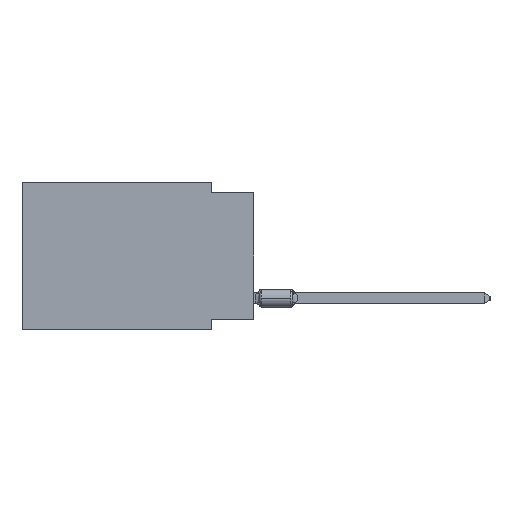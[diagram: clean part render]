
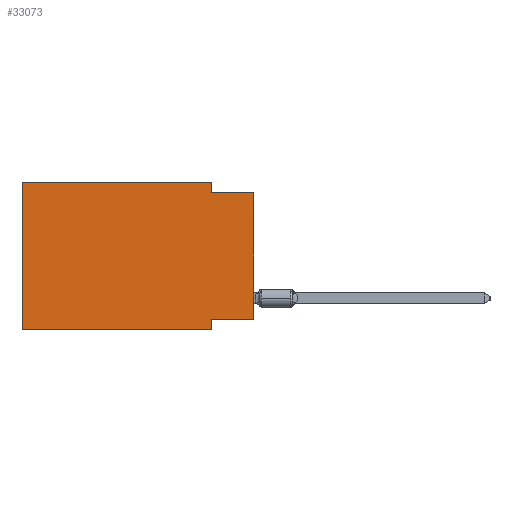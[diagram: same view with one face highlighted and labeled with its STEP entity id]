
A CAD part, left-side view. The second image highlights one B-rep face of the part: STEP entity #33073.
In plain terms, the highlighted planar face has unit normal (-1, 0, 0).
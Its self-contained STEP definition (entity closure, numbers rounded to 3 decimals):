
#757 = DIRECTION ( 'NONE',  ( 0., -1., 0. ) ) ;
#990 = CARTESIAN_POINT ( 'NONE',  ( 0., 0., -0.635 ) ) ;
#1292 = ORIENTED_EDGE ( 'NONE', *, *, #31722, .F. ) ;
#3122 = CARTESIAN_POINT ( 'NONE',  ( 0., 13.97, 0. ) ) ;
#3251 = DIRECTION ( 'NONE',  ( 0., 0., -1. ) ) ;
#3749 = VECTOR ( 'NONE', #3251, 1000. ) ;
#4054 = DIRECTION ( 'NONE',  ( 0., 0., 1. ) ) ;
#5217 = DIRECTION ( 'NONE',  ( 0., -1., 0. ) ) ;
#5792 = DIRECTION ( 'NONE',  ( 0., 0., -1. ) ) ;
#6641 = LINE ( 'NONE', #9706, #14677 ) ;
#6836 = CARTESIAN_POINT ( 'NONE',  ( 0., 2.54, 0. ) ) ;
#6910 = VERTEX_POINT ( 'NONE', #21703 ) ;
#7301 = DIRECTION ( 'NONE',  ( 0., 0., -1. ) ) ;
#7713 = CARTESIAN_POINT ( 'NONE',  ( 0., 2.54, -8.89 ) ) ;
#8044 = EDGE_CURVE ( 'NONE', #12465, #13004, #29062, .T. ) ;
#8526 = DIRECTION ( 'NONE',  ( 0., -1., 0. ) ) ;
#9296 = VECTOR ( 'NONE', #757, 1000. ) ;
#9335 = CARTESIAN_POINT ( 'NONE',  ( 0., 13.97, 0. ) ) ;
#9338 = VERTEX_POINT ( 'NONE', #39653 ) ;
#9567 = CARTESIAN_POINT ( 'NONE',  ( 0., 2.54, 0. ) ) ;
#9706 = CARTESIAN_POINT ( 'NONE',  ( 0., 0., -8.255 ) ) ;
#11923 = ORIENTED_EDGE ( 'NONE', *, *, #25752, .F. ) ;
#12383 = ORIENTED_EDGE ( 'NONE', *, *, #12802, .F. ) ;
#12465 = VERTEX_POINT ( 'NONE', #39825 ) ;
#12802 = EDGE_CURVE ( 'NONE', #9338, #14344, #18124, .T. ) ;
#13004 = VERTEX_POINT ( 'NONE', #26580 ) ;
#14344 = VERTEX_POINT ( 'NONE', #19650 ) ;
#14677 = VECTOR ( 'NONE', #27879, 1000. ) ;
#14922 = VECTOR ( 'NONE', #4054, 1000. ) ;
#15615 = CARTESIAN_POINT ( 'NONE',  ( 0., 13.97, -8.89 ) ) ;
#17947 = ORIENTED_EDGE ( 'NONE', *, *, #23432, .F. ) ;
#18124 = LINE ( 'NONE', #7713, #3749 ) ;
#18371 = ORIENTED_EDGE ( 'NONE', *, *, #41798, .F. ) ;
#19650 = CARTESIAN_POINT ( 'NONE',  ( 0., 2.54, -8.89 ) ) ;
#20772 = AXIS2_PLACEMENT_3D ( 'NONE', #9335, #37853, #5792 ) ;
#21625 = VECTOR ( 'NONE', #5217, 1000. ) ;
#21703 = CARTESIAN_POINT ( 'NONE',  ( 0., 0., -0.635 ) ) ;
#21821 = CARTESIAN_POINT ( 'NONE',  ( 0., 2.54, -0.635 ) ) ;
#21951 = EDGE_CURVE ( 'NONE', #42552, #6910, #26047, .T. ) ;
#22240 = LINE ( 'NONE', #15615, #9296 ) ;
#23432 = EDGE_CURVE ( 'NONE', #40999, #6910, #32838, .T. ) ;
#25019 = VERTEX_POINT ( 'NONE', #9567 ) ;
#25240 = LINE ( 'NONE', #6836, #35665 ) ;
#25752 = EDGE_CURVE ( 'NONE', #13004, #25019, #34215, .T. ) ;
#26047 = LINE ( 'NONE', #44627, #27289 ) ;
#26580 = CARTESIAN_POINT ( 'NONE',  ( 0., 13.97, 0. ) ) ;
#26696 = ORIENTED_EDGE ( 'NONE', *, *, #45926, .T. ) ;
#26736 = DIRECTION ( 'NONE',  ( 0., 0., 1. ) ) ;
#27162 = CARTESIAN_POINT ( 'NONE',  ( 0., 13.97, 0. ) ) ;
#27289 = VECTOR ( 'NONE', #26736, 1000. ) ;
#27879 = DIRECTION ( 'NONE',  ( 0., 1., 0. ) ) ;
#28379 = CARTESIAN_POINT ( 'NONE',  ( 0., 0., -8.255 ) ) ;
#29062 = LINE ( 'NONE', #3122, #14922 ) ;
#30347 = FACE_OUTER_BOUND ( 'NONE', #41518, .T. ) ;
#30799 = PLANE ( 'NONE',  #20772 ) ;
#31165 = VECTOR ( 'NONE', #8526, 1000. ) ;
#31722 = EDGE_CURVE ( 'NONE', #42552, #9338, #6641, .T. ) ;
#32838 = LINE ( 'NONE', #990, #31165 ) ;
#33073 = ADVANCED_FACE ( 'NONE', ( #30347 ), #30799, .F. ) ;
#34215 = LINE ( 'NONE', #27162, #21625 ) ;
#35665 = VECTOR ( 'NONE', #7301, 1000. ) ;
#37853 = DIRECTION ( 'NONE',  ( 1., 0., 0. ) ) ;
#38673 = ORIENTED_EDGE ( 'NONE', *, *, #21951, .T. ) ;
#39653 = CARTESIAN_POINT ( 'NONE',  ( 0., 2.54, -8.255 ) ) ;
#39825 = CARTESIAN_POINT ( 'NONE',  ( 0., 13.97, -8.89 ) ) ;
#39890 = ORIENTED_EDGE ( 'NONE', *, *, #8044, .F. ) ;
#40999 = VERTEX_POINT ( 'NONE', #21821 ) ;
#41518 = EDGE_LOOP ( 'NONE', ( #38673, #17947, #18371, #11923, #39890, #26696, #12383, #1292 ) ) ;
#41798 = EDGE_CURVE ( 'NONE', #25019, #40999, #25240, .T. ) ;
#42552 = VERTEX_POINT ( 'NONE', #28379 ) ;
#44627 = CARTESIAN_POINT ( 'NONE',  ( 0., 0., 0. ) ) ;
#45926 = EDGE_CURVE ( 'NONE', #12465, #14344, #22240, .T. ) ;
